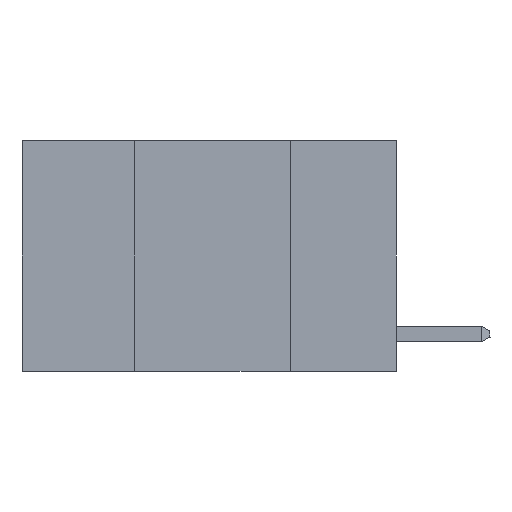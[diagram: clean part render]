
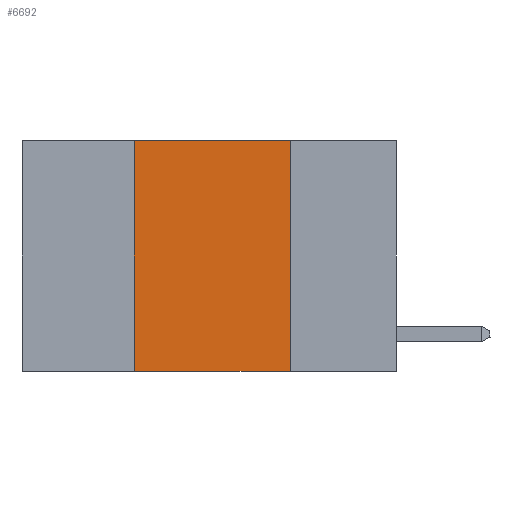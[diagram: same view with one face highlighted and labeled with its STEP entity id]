
A CAD part, left-side view. The second image highlights one B-rep face of the part: STEP entity #6692.
In plain terms, the highlighted planar face has unit normal (-1, 0, 0).
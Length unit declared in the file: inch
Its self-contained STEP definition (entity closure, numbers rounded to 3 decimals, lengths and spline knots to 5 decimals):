
#94 = LINE ( 'NONE', #7106, #10981 ) ;
#489 = ORIENTED_EDGE ( 'NONE', *, *, #13327, .F. ) ;
#527 = ORIENTED_EDGE ( 'NONE', *, *, #4671, .F. ) ;
#561 = ORIENTED_EDGE ( 'NONE', *, *, #7192, .F. ) ;
#587 = ORIENTED_EDGE ( 'NONE', *, *, #5683, .T. ) ;
#786 = CARTESIAN_POINT ( 'NONE',  ( 0., 0.17, 0. ) ) ;
#1218 = DIRECTION ( 'NONE',  ( 0., 0., -1. ) ) ;
#1346 = DIRECTION ( 'NONE',  ( 0., -1., 0. ) ) ;
#2000 = CARTESIAN_POINT ( 'NONE',  ( 0., 0.17, -0.37 ) ) ;
#3355 = CARTESIAN_POINT ( 'NONE',  ( 0., 0.17, 0. ) ) ;
#3470 = DIRECTION ( 'NONE',  ( 0., 0., 1. ) ) ;
#3655 = VECTOR ( 'NONE', #7457, 39.37008 ) ;
#4644 = CARTESIAN_POINT ( 'NONE',  ( 0., 0.6, 0. ) ) ;
#4671 = EDGE_CURVE ( 'NONE', #6218, #7729, #9534, .T. ) ;
#4704 = CARTESIAN_POINT ( 'NONE',  ( 0., 0.42, 0. ) ) ;
#5683 = EDGE_CURVE ( 'NONE', #7798, #12738, #94, .T. ) ;
#6218 = VERTEX_POINT ( 'NONE', #4704 ) ;
#6692 = ADVANCED_FACE ( 'NONE', ( #12752 ), #11283, .F. ) ;
#7106 = CARTESIAN_POINT ( 'NONE',  ( 0., 0.6, -0.37 ) ) ;
#7192 = EDGE_CURVE ( 'NONE', #7798, #6218, #7953, .T. ) ;
#7457 = DIRECTION ( 'NONE',  ( 0., -1., 0. ) ) ;
#7729 = VERTEX_POINT ( 'NONE', #3355 ) ;
#7798 = VERTEX_POINT ( 'NONE', #12160 ) ;
#7953 = LINE ( 'NONE', #8999, #10462 ) ;
#8027 = DIRECTION ( 'NONE',  ( 1., 0., 0. ) ) ;
#8549 = CARTESIAN_POINT ( 'NONE',  ( 0., 0.6, 0. ) ) ;
#8730 = DIRECTION ( 'NONE',  ( 0., 0., -1. ) ) ;
#8999 = CARTESIAN_POINT ( 'NONE',  ( 0., 0.42, 0. ) ) ;
#9081 = EDGE_LOOP ( 'NONE', ( #489, #527, #561, #587 ) ) ;
#9441 = AXIS2_PLACEMENT_3D ( 'NONE', #4644, #8027, #1218 ) ;
#9534 = LINE ( 'NONE', #8549, #3655 ) ;
#10462 = VECTOR ( 'NONE', #3470, 39.37008 ) ;
#10981 = VECTOR ( 'NONE', #1346, 39.37008 ) ;
#11283 = PLANE ( 'NONE',  #9441 ) ;
#11517 = VECTOR ( 'NONE', #8730, 39.37008 ) ;
#12160 = CARTESIAN_POINT ( 'NONE',  ( 0., 0.42, -0.37 ) ) ;
#12738 = VERTEX_POINT ( 'NONE', #2000 ) ;
#12752 = FACE_OUTER_BOUND ( 'NONE', #9081, .T. ) ;
#13327 = EDGE_CURVE ( 'NONE', #7729, #12738, #14259, .T. ) ;
#14259 = LINE ( 'NONE', #786, #11517 ) ;
